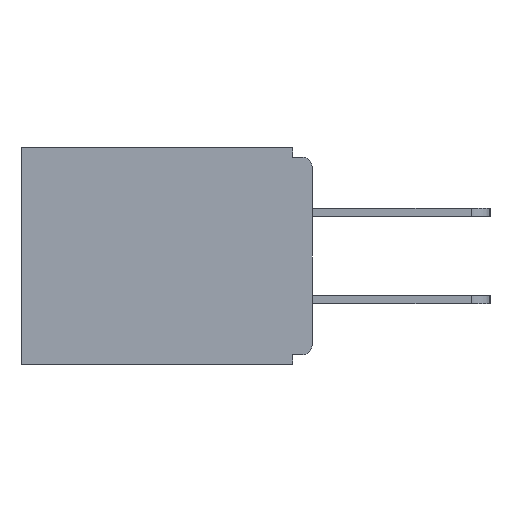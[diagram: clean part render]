
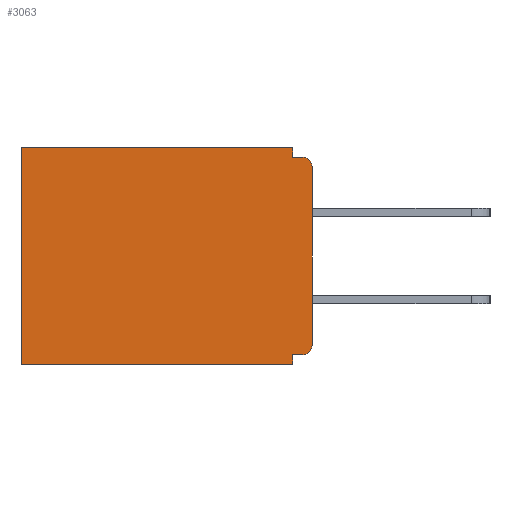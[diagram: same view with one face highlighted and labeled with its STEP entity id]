
A CAD part, left-side view. The second image highlights one B-rep face of the part: STEP entity #3063.
In plain terms, the highlighted planar face has unit normal (-1, 0, 0).
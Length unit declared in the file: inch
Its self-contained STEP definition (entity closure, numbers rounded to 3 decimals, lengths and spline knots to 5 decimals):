
#430 = CIRCLE ( 'NONE', #5280, 0.015 ) ;
#688 = VECTOR ( 'NONE', #1775, 39.37008 ) ;
#734 = CARTESIAN_POINT ( 'NONE',  ( 0.298, 0., -0.328 ) ) ;
#856 = ORIENTED_EDGE ( 'NONE', *, *, #6045, .F. ) ;
#1099 = ORIENTED_EDGE ( 'NONE', *, *, #6038, .F. ) ;
#1251 = DIRECTION ( 'NONE',  ( 0., 1., 0. ) ) ;
#1445 = ORIENTED_EDGE ( 'NONE', *, *, #16319, .F. ) ;
#1775 = DIRECTION ( 'NONE',  ( 0., -1., 0. ) ) ;
#2106 = LINE ( 'NONE', #5147, #13781 ) ;
#2350 = ORIENTED_EDGE ( 'NONE', *, *, #12646, .T. ) ;
#2559 = ORIENTED_EDGE ( 'NONE', *, *, #9515, .F. ) ;
#2563 = VERTEX_POINT ( 'NONE', #5504 ) ;
#2647 = LINE ( 'NONE', #10875, #6784 ) ;
#3063 = ADVANCED_FACE ( 'NONE', ( #7274 ), #3377, .F. ) ;
#3150 = DIRECTION ( 'NONE',  ( 1., 0., 0. ) ) ;
#3316 = LINE ( 'NONE', #12731, #14776 ) ;
#3377 = PLANE ( 'NONE',  #14856 ) ;
#3526 = EDGE_CURVE ( 'NONE', #10372, #6491, #7856, .T. ) ;
#3649 = EDGE_CURVE ( 'NONE', #5199, #12153, #6255, .T. ) ;
#3718 = CARTESIAN_POINT ( 'NONE',  ( 0.298, 0., -0.313 ) ) ;
#3845 = LINE ( 'NONE', #734, #4595 ) ;
#4595 = VECTOR ( 'NONE', #5826, 39.37008 ) ;
#4749 = CARTESIAN_POINT ( 'NONE',  ( 0.298, 0.015, -0.015 ) ) ;
#5110 = CARTESIAN_POINT ( 'NONE',  ( 0.298, 0.015, -0.313 ) ) ;
#5130 = CARTESIAN_POINT ( 'NONE',  ( 0.298, 0.015, -0.03 ) ) ;
#5147 = CARTESIAN_POINT ( 'NONE',  ( 0.298, 0., 0. ) ) ;
#5199 = VERTEX_POINT ( 'NONE', #10971 ) ;
#5280 = AXIS2_PLACEMENT_3D ( 'NONE', #5110, #15264, #7662 ) ;
#5504 = CARTESIAN_POINT ( 'NONE',  ( 0.298, 0.015, -0.328 ) ) ;
#5714 = ORIENTED_EDGE ( 'NONE', *, *, #14145, .T. ) ;
#5726 = ORIENTED_EDGE ( 'NONE', *, *, #5837, .F. ) ;
#5826 = DIRECTION ( 'NONE',  ( 0., 1., 0. ) ) ;
#5837 = EDGE_CURVE ( 'NONE', #6673, #6491, #8992, .T. ) ;
#6038 = EDGE_CURVE ( 'NONE', #2563, #14818, #3845, .T. ) ;
#6045 = EDGE_CURVE ( 'NONE', #14818, #5199, #2647, .T. ) ;
#6255 = LINE ( 'NONE', #16200, #7247 ) ;
#6284 = EDGE_LOOP ( 'NONE', ( #13499, #5726, #2559, #7001, #5714, #6427, #856, #1099, #2350, #1445 ) ) ;
#6363 = AXIS2_PLACEMENT_3D ( 'NONE', #5130, #12814, #12922 ) ;
#6427 = ORIENTED_EDGE ( 'NONE', *, *, #3649, .F. ) ;
#6491 = VERTEX_POINT ( 'NONE', #4749 ) ;
#6673 = VERTEX_POINT ( 'NONE', #7674 ) ;
#6681 = CARTESIAN_POINT ( 'NONE',  ( 0.298, 0., -0.015 ) ) ;
#6784 = VECTOR ( 'NONE', #10935, 39.37008 ) ;
#6951 = DIRECTION ( 'NONE',  ( 0., 0., -1. ) ) ;
#7001 = ORIENTED_EDGE ( 'NONE', *, *, #9884, .T. ) ;
#7091 = DIRECTION ( 'NONE',  ( 0., 0., -1. ) ) ;
#7194 = CARTESIAN_POINT ( 'NONE',  ( 0.298, 0.46, 0. ) ) ;
#7247 = VECTOR ( 'NONE', #1251, 39.37008 ) ;
#7274 = FACE_OUTER_BOUND ( 'NONE', #6284, .T. ) ;
#7521 = DIRECTION ( 'NONE',  ( 0., 1., 0. ) ) ;
#7524 = VERTEX_POINT ( 'NONE', #15739 ) ;
#7662 = DIRECTION ( 'NONE',  ( 0., 0., -1. ) ) ;
#7674 = CARTESIAN_POINT ( 'NONE',  ( 0.298, 0.031, -0.015 ) ) ;
#7787 = CARTESIAN_POINT ( 'NONE',  ( 0.298, 0.46, -0.343 ) ) ;
#7856 = CIRCLE ( 'NONE', #6363, 0.015 ) ;
#7916 = VECTOR ( 'NONE', #7091, 39.37008 ) ;
#8567 = LINE ( 'NONE', #7194, #11587 ) ;
#8992 = LINE ( 'NONE', #6681, #688 ) ;
#9515 = EDGE_CURVE ( 'NONE', #7524, #6673, #3316, .T. ) ;
#9685 = CARTESIAN_POINT ( 'NONE',  ( 0.298, 0.46, 0. ) ) ;
#9726 = CARTESIAN_POINT ( 'NONE',  ( 0.298, 0., 0. ) ) ;
#9884 = EDGE_CURVE ( 'NONE', #7524, #10522, #2106, .T. ) ;
#10372 = VERTEX_POINT ( 'NONE', #11392 ) ;
#10522 = VERTEX_POINT ( 'NONE', #9685 ) ;
#10813 = CARTESIAN_POINT ( 'NONE',  ( 0.298, 0., 0. ) ) ;
#10875 = CARTESIAN_POINT ( 'NONE',  ( 0.298, 0.031, -0.343 ) ) ;
#10935 = DIRECTION ( 'NONE',  ( 0., 0., -1. ) ) ;
#10971 = CARTESIAN_POINT ( 'NONE',  ( 0.298, 0.031, -0.343 ) ) ;
#11290 = DIRECTION ( 'NONE',  ( 0., 0., -1. ) ) ;
#11392 = CARTESIAN_POINT ( 'NONE',  ( 0.298, 0., -0.03 ) ) ;
#11587 = VECTOR ( 'NONE', #11290, 39.37008 ) ;
#12085 = VERTEX_POINT ( 'NONE', #3718 ) ;
#12153 = VERTEX_POINT ( 'NONE', #7787 ) ;
#12646 = EDGE_CURVE ( 'NONE', #2563, #12085, #430, .T. ) ;
#12731 = CARTESIAN_POINT ( 'NONE',  ( 0.298, 0.031, -0.343 ) ) ;
#12814 = DIRECTION ( 'NONE',  ( -1., 0., 0. ) ) ;
#12835 = CARTESIAN_POINT ( 'NONE',  ( 0.298, 0.031, -0.328 ) ) ;
#12922 = DIRECTION ( 'NONE',  ( 0., 0., -1. ) ) ;
#13267 = LINE ( 'NONE', #10813, #7916 ) ;
#13499 = ORIENTED_EDGE ( 'NONE', *, *, #3526, .T. ) ;
#13781 = VECTOR ( 'NONE', #7521, 39.37008 ) ;
#14037 = DIRECTION ( 'NONE',  ( 0., 0., -1. ) ) ;
#14145 = EDGE_CURVE ( 'NONE', #10522, #12153, #8567, .T. ) ;
#14776 = VECTOR ( 'NONE', #14037, 39.37008 ) ;
#14818 = VERTEX_POINT ( 'NONE', #12835 ) ;
#14856 = AXIS2_PLACEMENT_3D ( 'NONE', #9726, #3150, #6951 ) ;
#15264 = DIRECTION ( 'NONE',  ( -1., 0., 0. ) ) ;
#15739 = CARTESIAN_POINT ( 'NONE',  ( 0.298, 0.031, 0. ) ) ;
#16200 = CARTESIAN_POINT ( 'NONE',  ( 0.298, 0., -0.343 ) ) ;
#16319 = EDGE_CURVE ( 'NONE', #10372, #12085, #13267, .T. ) ;
